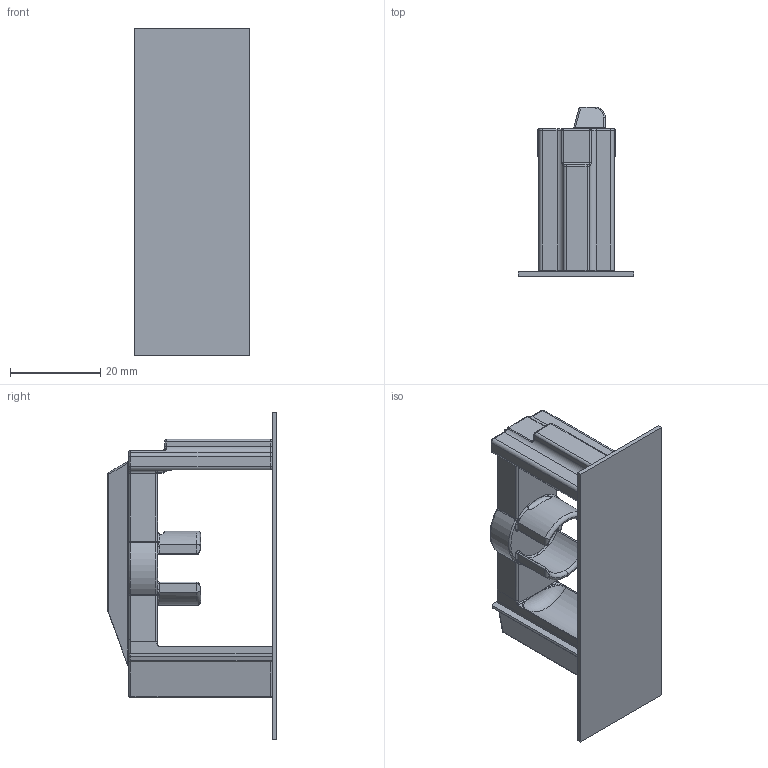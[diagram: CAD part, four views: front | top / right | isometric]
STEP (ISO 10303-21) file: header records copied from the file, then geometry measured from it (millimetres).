
FILE_DESCRIPTION(/* description */ ('STEP AP214'),/* implementation_level */ '2;1');
FILE_NAME(/* name */ 'Ivan''Ivan''s Standard Follower.stp',/* time_stamp */ '2019-01-27T20:56:03-06:00',/* author */ ('johne'),/* organization */ (''),/* preprocessor_version */ 'ST-DEVELOPER v16.13',/* originating_system */ 'Autodesk Inventor 2018',/* authorisation */ '');
FILE_SCHEMA (('AUTOMOTIVE_DESIGN { 1 0 10303 214 3 1 1 }'));
Length unit declared in the file: millimetre
Products named in the file (1): DefDist_Cuomo_AR15_30_Mag_Follower
Bounding box: 25.54 x 37.53 x 72.6 mm (x, y, z)
Volume: 10818.2 mm3; surface area: 10312.8 mm2
Topology: 1 solids, 1 shells, 314 faces, 775 edges, 446 vertices
Faces by surface type: cylinder 118, bspline 67, torus 64, plane 56, sphere 9
Full cylindrical faces by diameter (mm): 2.388 x1
Entity records: 14411 total; most frequent: CARTESIAN_POINT 7348, ORIENTED_EDGE 1506, DIRECTION 1472, EDGE_CURVE 753, AXIS2_PLACEMENT_3D 601, VERTEX_POINT 444, EDGE_LOOP 317, FACE_OUTER_BOUND 312
